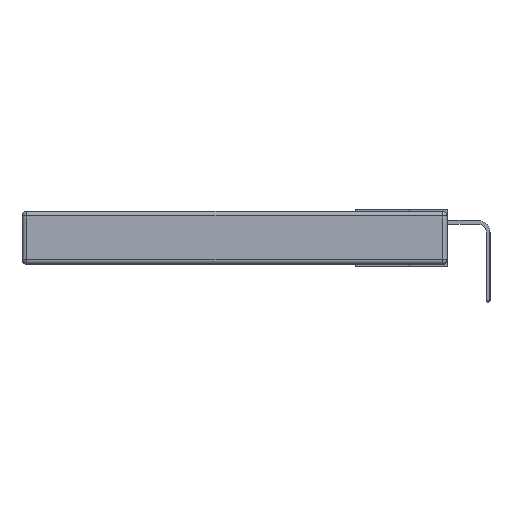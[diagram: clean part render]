
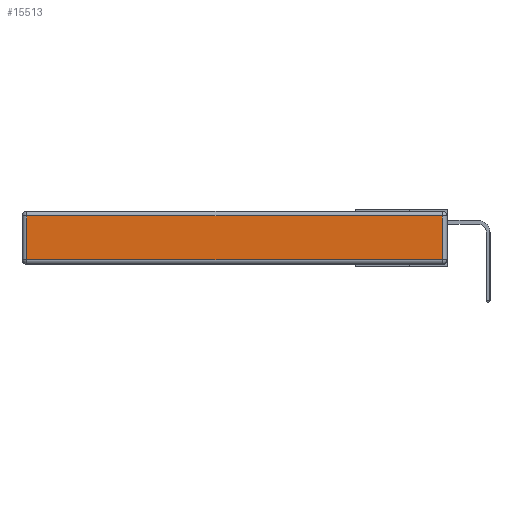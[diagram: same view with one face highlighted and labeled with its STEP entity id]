
A CAD part, left-side view. The second image highlights one B-rep face of the part: STEP entity #15513.
In plain terms, the highlighted planar face has unit normal (-1, 0, 0).
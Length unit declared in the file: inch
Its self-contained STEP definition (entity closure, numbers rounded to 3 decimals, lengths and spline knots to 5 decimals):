
#431 = ORIENTED_EDGE ( 'NONE', *, *, #9073, .T. ) ;
#827 = ORIENTED_EDGE ( 'NONE', *, *, #1425, .T. ) ;
#1349 = VECTOR ( 'NONE', #2752, 39.37008 ) ;
#1425 = EDGE_CURVE ( 'NONE', #5744, #14859, #2508, .T. ) ;
#2098 = EDGE_CURVE ( 'NONE', #5530, #13301, #14003, .T. ) ;
#2195 = CARTESIAN_POINT ( 'NONE',  ( 0., 0., -0.313 ) ) ;
#2209 = DIRECTION ( 'NONE',  ( 0., 0., 1. ) ) ;
#2269 = PLANE ( 'NONE',  #5950 ) ;
#2508 = LINE ( 'NONE', #2195, #14273 ) ;
#2752 = DIRECTION ( 'NONE',  ( 0., 0., -1. ) ) ;
#3559 = EDGE_LOOP ( 'NONE', ( #827, #14296, #9186, #431 ) ) ;
#4032 = CARTESIAN_POINT ( 'NONE',  ( 0., 2.72, -0.343 ) ) ;
#5253 = LINE ( 'NONE', #4032, #1349 ) ;
#5381 = CARTESIAN_POINT ( 'NONE',  ( 0., 0.03, -0.343 ) ) ;
#5530 = VERTEX_POINT ( 'NONE', #14921 ) ;
#5744 = VERTEX_POINT ( 'NONE', #17270 ) ;
#5787 = LINE ( 'NONE', #5381, #7453 ) ;
#5950 = AXIS2_PLACEMENT_3D ( 'NONE', #6954, #6765, #2209 ) ;
#6708 = CARTESIAN_POINT ( 'NONE',  ( 0., 2.72, -0.03 ) ) ;
#6765 = DIRECTION ( 'NONE',  ( -1., 0., 0. ) ) ;
#6954 = CARTESIAN_POINT ( 'NONE',  ( 0., 0., -0.343 ) ) ;
#7426 = EDGE_CURVE ( 'NONE', #14859, #5530, #5787, .T. ) ;
#7453 = VECTOR ( 'NONE', #17650, 39.37008 ) ;
#7505 = VECTOR ( 'NONE', #9225, 39.37008 ) ;
#9073 = EDGE_CURVE ( 'NONE', #13301, #5744, #5253, .T. ) ;
#9186 = ORIENTED_EDGE ( 'NONE', *, *, #2098, .T. ) ;
#9225 = DIRECTION ( 'NONE',  ( 0., 1., 0. ) ) ;
#13301 = VERTEX_POINT ( 'NONE', #6708 ) ;
#14003 = LINE ( 'NONE', #18703, #7505 ) ;
#14273 = VECTOR ( 'NONE', #16386, 39.37008 ) ;
#14296 = ORIENTED_EDGE ( 'NONE', *, *, #7426, .T. ) ;
#14859 = VERTEX_POINT ( 'NONE', #17194 ) ;
#14921 = CARTESIAN_POINT ( 'NONE',  ( 0., 0.03, -0.03 ) ) ;
#15082 = FACE_OUTER_BOUND ( 'NONE', #3559, .T. ) ;
#15513 = ADVANCED_FACE ( 'NONE', ( #15082 ), #2269, .T. ) ;
#16386 = DIRECTION ( 'NONE',  ( 0., -1., 0. ) ) ;
#17194 = CARTESIAN_POINT ( 'NONE',  ( 0., 0.03, -0.313 ) ) ;
#17270 = CARTESIAN_POINT ( 'NONE',  ( 0., 2.72, -0.313 ) ) ;
#17650 = DIRECTION ( 'NONE',  ( 0., 0., 1. ) ) ;
#18703 = CARTESIAN_POINT ( 'NONE',  ( 0., 2.75, -0.03 ) ) ;
